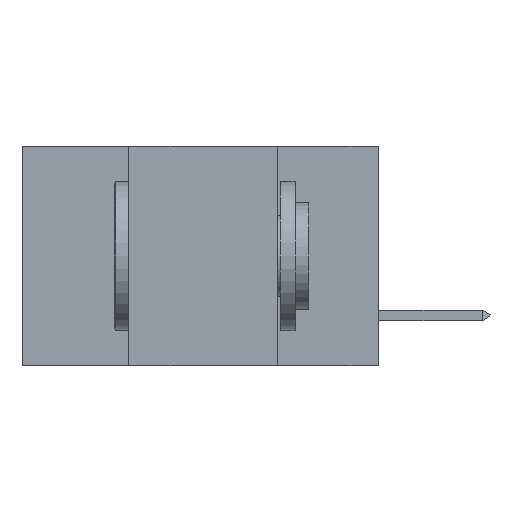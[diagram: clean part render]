
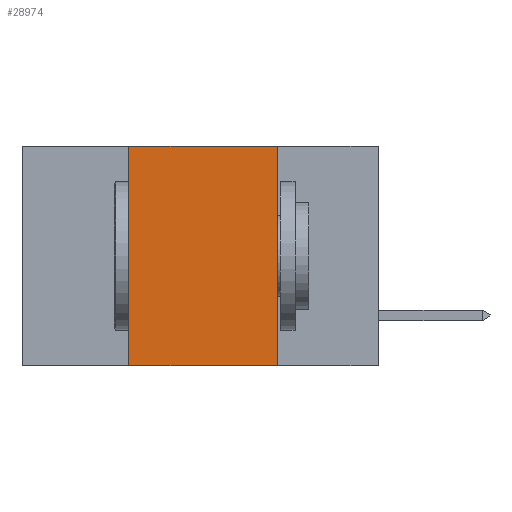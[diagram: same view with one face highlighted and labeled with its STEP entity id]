
A CAD part, left-side view. The second image highlights one B-rep face of the part: STEP entity #28974.
In plain terms, the highlighted planar face has unit normal (-1, 0, 0).
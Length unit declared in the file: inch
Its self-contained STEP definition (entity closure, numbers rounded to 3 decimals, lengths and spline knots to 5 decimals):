
#269 = ORIENTED_EDGE ( 'NONE', *, *, #16017, .F. ) ;
#311 = LINE ( 'NONE', #7075, #7166 ) ;
#1502 = CARTESIAN_POINT ( 'NONE',  ( 0., 0.42, -0.37 ) ) ;
#1593 = VECTOR ( 'NONE', #23893, 39.37008 ) ;
#3022 = ORIENTED_EDGE ( 'NONE', *, *, #8335, .F. ) ;
#3044 = CARTESIAN_POINT ( 'NONE',  ( 0., 0.6, 0. ) ) ;
#3247 = PLANE ( 'NONE',  #24201 ) ;
#3835 = CARTESIAN_POINT ( 'NONE',  ( 0., 0.42, 0. ) ) ;
#4722 = DIRECTION ( 'NONE',  ( 0., 0., -1. ) ) ;
#7075 = CARTESIAN_POINT ( 'NONE',  ( 0., 0.17, 0. ) ) ;
#7166 = VECTOR ( 'NONE', #4722, 39.37008 ) ;
#8335 = EDGE_CURVE ( 'NONE', #19204, #17903, #18185, .T. ) ;
#9230 = CARTESIAN_POINT ( 'NONE',  ( 0., 0.17, -0.37 ) ) ;
#9609 = LINE ( 'NONE', #23996, #1593 ) ;
#10469 = VERTEX_POINT ( 'NONE', #17201 ) ;
#13096 = ORIENTED_EDGE ( 'NONE', *, *, #13116, .F. ) ;
#13116 = EDGE_CURVE ( 'NONE', #17903, #10469, #9609, .T. ) ;
#14026 = VECTOR ( 'NONE', #27968, 39.37008 ) ;
#16017 = EDGE_CURVE ( 'NONE', #10469, #18451, #311, .T. ) ;
#17201 = CARTESIAN_POINT ( 'NONE',  ( 0., 0.17, 0. ) ) ;
#17903 = VERTEX_POINT ( 'NONE', #3835 ) ;
#18124 = DIRECTION ( 'NONE',  ( 0., -1., 0. ) ) ;
#18185 = LINE ( 'NONE', #22343, #14026 ) ;
#18451 = VERTEX_POINT ( 'NONE', #9230 ) ;
#19204 = VERTEX_POINT ( 'NONE', #1502 ) ;
#20671 = FACE_OUTER_BOUND ( 'NONE', #25632, .T. ) ;
#22208 = ORIENTED_EDGE ( 'NONE', *, *, #24542, .T. ) ;
#22343 = CARTESIAN_POINT ( 'NONE',  ( 0., 0.42, 0. ) ) ;
#23893 = DIRECTION ( 'NONE',  ( 0., -1., 0. ) ) ;
#23996 = CARTESIAN_POINT ( 'NONE',  ( 0., 0.6, 0. ) ) ;
#24201 = AXIS2_PLACEMENT_3D ( 'NONE', #3044, #27175, #25062 ) ;
#24542 = EDGE_CURVE ( 'NONE', #19204, #18451, #27052, .T. ) ;
#25062 = DIRECTION ( 'NONE',  ( 0., 0., -1. ) ) ;
#25632 = EDGE_LOOP ( 'NONE', ( #269, #13096, #3022, #22208 ) ) ;
#27052 = LINE ( 'NONE', #30108, #30111 ) ;
#27175 = DIRECTION ( 'NONE',  ( 1., 0., 0. ) ) ;
#27968 = DIRECTION ( 'NONE',  ( 0., 0., 1. ) ) ;
#28974 = ADVANCED_FACE ( 'NONE', ( #20671 ), #3247, .F. ) ;
#30108 = CARTESIAN_POINT ( 'NONE',  ( 0., 0.6, -0.37 ) ) ;
#30111 = VECTOR ( 'NONE', #18124, 39.37008 ) ;
